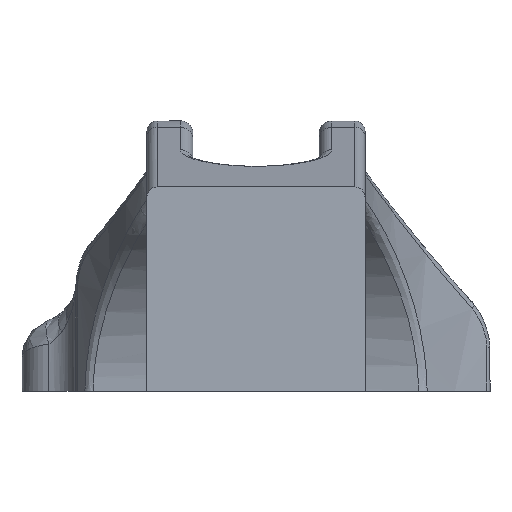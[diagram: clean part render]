
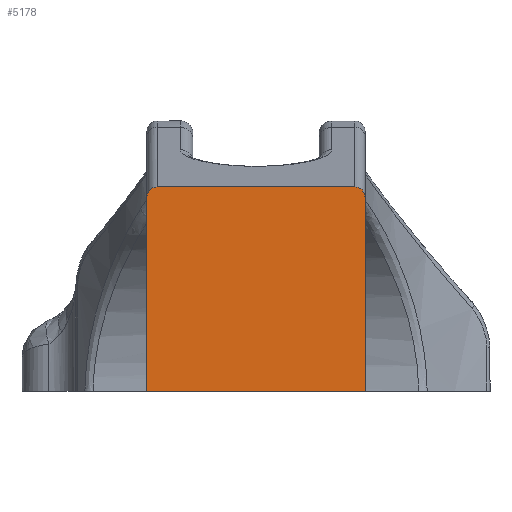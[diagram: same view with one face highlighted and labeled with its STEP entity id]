
A CAD part, front view. The second image highlights one B-rep face of the part: STEP entity #5178.
In plain terms, the highlighted planar face has unit normal (0, -1, 0).
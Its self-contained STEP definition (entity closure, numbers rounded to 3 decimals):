
#150 = VECTOR ( 'NONE', #5037, 1000. ) ;
#315 = LINE ( 'NONE', #1063, #2815 ) ;
#530 = VERTEX_POINT ( 'NONE', #4584 ) ;
#598 = CARTESIAN_POINT ( 'NONE',  ( 21.364, -48.289, 153.013 ) ) ;
#693 =( BOUNDED_CURVE ( )  B_SPLINE_CURVE ( 3, ( #5263, #835, #1839, #5280 ),
 .UNSPECIFIED., .F., .F. ) 
 B_SPLINE_CURVE_WITH_KNOTS ( ( 4, 4 ),
 ( 0., 1.571 ),
 .UNSPECIFIED. ) 
 CURVE ( )  GEOMETRIC_REPRESENTATION_ITEM ( )  RATIONAL_B_SPLINE_CURVE ( ( 1., 0.805, 0.805, 1. ) ) 
 REPRESENTATION_ITEM ( '' )  );
#698 = DIRECTION ( 'NONE',  ( 0., 0., -1. ) ) ;
#835 = CARTESIAN_POINT ( 'NONE',  ( 21.035, -48.289, 212.69 ) ) ;
#907 = ORIENTED_EDGE ( 'NONE', *, *, #3086, .T. ) ;
#1063 = CARTESIAN_POINT ( 'NONE',  ( 21.364, -48.289, 153.013 ) ) ;
#1088 = ORIENTED_EDGE ( 'NONE', *, *, #4111, .F. ) ;
#1399 = EDGE_CURVE ( 'NONE', #4372, #2362, #5215, .T. ) ;
#1492 = LINE ( 'NONE', #5248, #2846 ) ;
#1515 = AXIS2_PLACEMENT_3D ( 'NONE', #598, #3691, #698 ) ;
#1576 = EDGE_LOOP ( 'NONE', ( #5801, #907, #1088, #3377, #4577, #4719 ) ) ;
#1839 = CARTESIAN_POINT ( 'NONE',  ( 21.364, -48.289, 212.354 ) ) ;
#2252 = CARTESIAN_POINT ( 'NONE',  ( 21.364, -48.289, 196.492 ) ) ;
#2362 = VERTEX_POINT ( 'NONE', #2586 ) ;
#2459 = VECTOR ( 'NONE', #5374, 1000. ) ;
#2586 = CARTESIAN_POINT ( 'NONE',  ( 4.86, -48.289, 212.69 ) ) ;
#2795 = LINE ( 'NONE', #4917, #2459 ) ;
#2815 = VECTOR ( 'NONE', #4048, 1000. ) ;
#2817 = DIRECTION ( 'NONE',  ( 0., 0., 1. ) ) ;
#2846 = VECTOR ( 'NONE', #2817, 1000. ) ;
#3086 = EDGE_CURVE ( 'NONE', #3930, #530, #315, .T. ) ;
#3095 = EDGE_CURVE ( 'NONE', #2362, #6010, #4126, .T. ) ;
#3377 = ORIENTED_EDGE ( 'NONE', *, *, #3095, .F. ) ;
#3535 = EDGE_CURVE ( 'NONE', #5845, #4372, #1492, .T. ) ;
#3691 = DIRECTION ( 'NONE',  ( 0., 1., 0. ) ) ;
#3930 = VERTEX_POINT ( 'NONE', #2252 ) ;
#4048 = DIRECTION ( 'NONE',  ( 0., 0., 1. ) ) ;
#4111 = EDGE_CURVE ( 'NONE', #6010, #530, #693, .T. ) ;
#4126 = LINE ( 'NONE', #4555, #150 ) ;
#4372 = VERTEX_POINT ( 'NONE', #5851 ) ;
#4555 = CARTESIAN_POINT ( 'NONE',  ( 21.364, -48.289, 212.69 ) ) ;
#4577 = ORIENTED_EDGE ( 'NONE', *, *, #1399, .F. ) ;
#4584 = CARTESIAN_POINT ( 'NONE',  ( 21.364, -48.289, 211.877 ) ) ;
#4719 = ORIENTED_EDGE ( 'NONE', *, *, #3535, .F. ) ;
#4917 = CARTESIAN_POINT ( 'NONE',  ( -9.788, -48.289, 196.492 ) ) ;
#4967 = EDGE_CURVE ( 'NONE', #5845, #3930, #2795, .T. ) ;
#5037 = DIRECTION ( 'NONE',  ( 1., 0., 0. ) ) ;
#5058 = CARTESIAN_POINT ( 'NONE',  ( 4.86, -48.289, 212.69 ) ) ;
#5070 = PLANE ( 'NONE',  #1515 ) ;
#5086 = CARTESIAN_POINT ( 'NONE',  ( 4.067, -48.289, 211.877 ) ) ;
#5101 = CARTESIAN_POINT ( 'NONE',  ( 4.067, -48.289, 212.354 ) ) ;
#5127 = CARTESIAN_POINT ( 'NONE',  ( 4.396, -48.289, 212.69 ) ) ;
#5178 = ADVANCED_FACE ( 'NONE', ( #5876 ), #5070, .F. ) ;
#5184 = CARTESIAN_POINT ( 'NONE',  ( 20.57, -48.289, 212.69 ) ) ;
#5215 =( BOUNDED_CURVE ( )  B_SPLINE_CURVE ( 3, ( #5086, #5101, #5127, #5058 ),
 .UNSPECIFIED., .F., .F. ) 
 B_SPLINE_CURVE_WITH_KNOTS ( ( 4, 4 ),
 ( 1.571, 3.142 ),
 .UNSPECIFIED. ) 
 CURVE ( )  GEOMETRIC_REPRESENTATION_ITEM ( )  RATIONAL_B_SPLINE_CURVE ( ( 1., 0.805, 0.805, 1. ) ) 
 REPRESENTATION_ITEM ( '' )  );
#5248 = CARTESIAN_POINT ( 'NONE',  ( 4.067, -48.289, 153.013 ) ) ;
#5263 = CARTESIAN_POINT ( 'NONE',  ( 20.57, -48.289, 212.69 ) ) ;
#5280 = CARTESIAN_POINT ( 'NONE',  ( 21.364, -48.289, 211.877 ) ) ;
#5374 = DIRECTION ( 'NONE',  ( 1., 0., 0. ) ) ;
#5801 = ORIENTED_EDGE ( 'NONE', *, *, #4967, .T. ) ;
#5845 = VERTEX_POINT ( 'NONE', #6055 ) ;
#5851 = CARTESIAN_POINT ( 'NONE',  ( 4.067, -48.289, 211.877 ) ) ;
#5876 = FACE_OUTER_BOUND ( 'NONE', #1576, .T. ) ;
#6010 = VERTEX_POINT ( 'NONE', #5184 ) ;
#6055 = CARTESIAN_POINT ( 'NONE',  ( 4.067, -48.289, 196.492 ) ) ;
